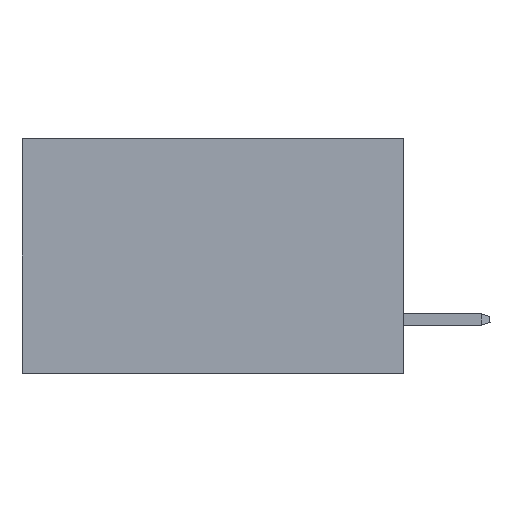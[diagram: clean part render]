
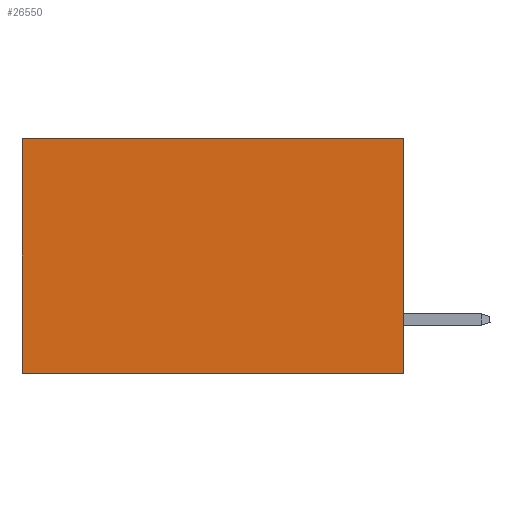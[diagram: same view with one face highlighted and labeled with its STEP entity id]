
A CAD part, left-side view. The second image highlights one B-rep face of the part: STEP entity #26550.
In plain terms, the highlighted planar face has unit normal (-1, 0, 0).
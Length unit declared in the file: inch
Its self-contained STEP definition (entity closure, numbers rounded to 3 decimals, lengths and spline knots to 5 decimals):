
#1981 = ORIENTED_EDGE ( 'NONE', *, *, #31665, .T. ) ;
#4311 = LINE ( 'NONE', #26741, #26802 ) ;
#6830 = CARTESIAN_POINT ( 'NONE',  ( 0.2875, 0.6, -0.37 ) ) ;
#6959 = ORIENTED_EDGE ( 'NONE', *, *, #21221, .F. ) ;
#9331 = DIRECTION ( 'NONE',  ( 1., 0., 0. ) ) ;
#10663 = VECTOR ( 'NONE', #11053, 39.37008 ) ;
#10721 = VERTEX_POINT ( 'NONE', #6830 ) ;
#11053 = DIRECTION ( 'NONE',  ( 0., 0., -1. ) ) ;
#11821 = EDGE_LOOP ( 'NONE', ( #31755, #26855, #6959, #1981 ) ) ;
#11903 = CARTESIAN_POINT ( 'NONE',  ( 0.2875, 0., 0. ) ) ;
#12438 = FACE_OUTER_BOUND ( 'NONE', #11821, .T. ) ;
#13738 = CARTESIAN_POINT ( 'NONE',  ( 0.2875, 0.6, 0. ) ) ;
#16612 = CARTESIAN_POINT ( 'NONE',  ( 0.2875, 0., 0. ) ) ;
#16812 = CARTESIAN_POINT ( 'NONE',  ( 0.2875, 0., 0. ) ) ;
#19337 = CARTESIAN_POINT ( 'NONE',  ( 0.2875, 0.6, 0. ) ) ;
#19757 = VERTEX_POINT ( 'NONE', #13738 ) ;
#19852 = VECTOR ( 'NONE', #33922, 39.37008 ) ;
#20064 = LINE ( 'NONE', #19337, #10663 ) ;
#20643 = EDGE_CURVE ( 'NONE', #19757, #10721, #20064, .T. ) ;
#21221 = EDGE_CURVE ( 'NONE', #35612, #22479, #28832, .T. ) ;
#21453 = AXIS2_PLACEMENT_3D ( 'NONE', #23654, #9331, #35060 ) ;
#22479 = VERTEX_POINT ( 'NONE', #25791 ) ;
#23122 = DIRECTION ( 'NONE',  ( 0., 0., -1. ) ) ;
#23654 = CARTESIAN_POINT ( 'NONE',  ( 0.2875, 0., 0. ) ) ;
#25791 = CARTESIAN_POINT ( 'NONE',  ( 0.2875, 0., -0.37 ) ) ;
#26550 = ADVANCED_FACE ( 'NONE', ( #12438 ), #29002, .F. ) ;
#26551 = VECTOR ( 'NONE', #23122, 39.37008 ) ;
#26741 = CARTESIAN_POINT ( 'NONE',  ( 0.2875, 0., -0.37 ) ) ;
#26802 = VECTOR ( 'NONE', #29317, 39.37008 ) ;
#26855 = ORIENTED_EDGE ( 'NONE', *, *, #34218, .F. ) ;
#28832 = LINE ( 'NONE', #11903, #26551 ) ;
#29002 = PLANE ( 'NONE',  #21453 ) ;
#29317 = DIRECTION ( 'NONE',  ( 0., 1., 0. ) ) ;
#31338 = LINE ( 'NONE', #16812, #19852 ) ;
#31665 = EDGE_CURVE ( 'NONE', #35612, #19757, #31338, .T. ) ;
#31755 = ORIENTED_EDGE ( 'NONE', *, *, #20643, .T. ) ;
#33922 = DIRECTION ( 'NONE',  ( 0., 1., 0. ) ) ;
#34218 = EDGE_CURVE ( 'NONE', #22479, #10721, #4311, .T. ) ;
#35060 = DIRECTION ( 'NONE',  ( 0., 0., -1. ) ) ;
#35612 = VERTEX_POINT ( 'NONE', #16612 ) ;
